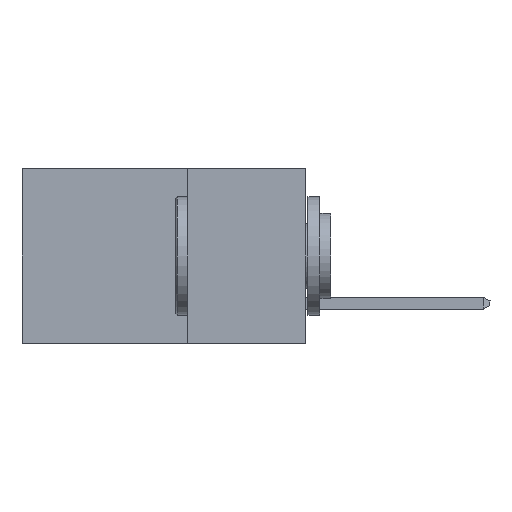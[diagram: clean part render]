
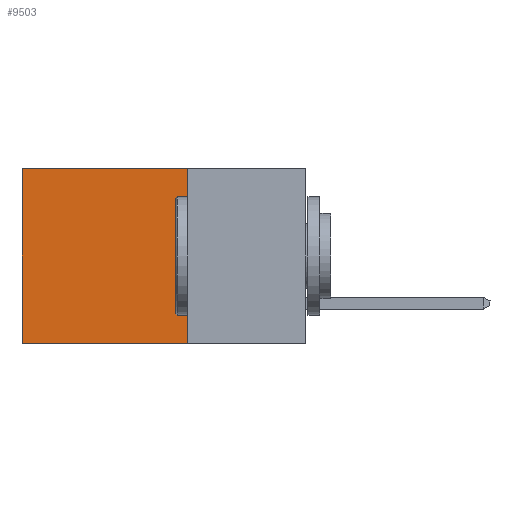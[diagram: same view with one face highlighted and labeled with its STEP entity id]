
A CAD part, left-side view. The second image highlights one B-rep face of the part: STEP entity #9503.
In plain terms, the highlighted planar face has unit normal (-1, 0, 0).
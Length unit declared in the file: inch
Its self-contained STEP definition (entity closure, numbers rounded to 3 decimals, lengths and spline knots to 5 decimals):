
#508 = EDGE_CURVE ( 'NONE', #12807, #16303, #17546, .T. ) ;
#729 = LINE ( 'NONE', #22717, #8557 ) ;
#1144 = DIRECTION ( 'NONE',  ( 1., 0., 0. ) ) ;
#1197 = ORIENTED_EDGE ( 'NONE', *, *, #27011, .F. ) ;
#1852 = CARTESIAN_POINT ( 'NONE',  ( 0.298, 0.25, 0. ) ) ;
#2166 = ORIENTED_EDGE ( 'NONE', *, *, #22689, .F. ) ;
#2172 = VECTOR ( 'NONE', #9424, 39.37008 ) ;
#3551 = CARTESIAN_POINT ( 'NONE',  ( 0.298, 0.25, 0. ) ) ;
#4534 = EDGE_LOOP ( 'NONE', ( #17804, #1197, #2166, #8695 ) ) ;
#5221 = LINE ( 'NONE', #24693, #2172 ) ;
#5830 = PLANE ( 'NONE',  #9291 ) ;
#8433 = LINE ( 'NONE', #10832, #19733 ) ;
#8557 = VECTOR ( 'NONE', #20531, 39.37008 ) ;
#8695 = ORIENTED_EDGE ( 'NONE', *, *, #508, .T. ) ;
#9291 = AXIS2_PLACEMENT_3D ( 'NONE', #3551, #1144, #12366 ) ;
#9424 = DIRECTION ( 'NONE',  ( 0., 0., -1. ) ) ;
#9503 = ADVANCED_FACE ( 'NONE', ( #22733 ), #5830, .F. ) ;
#10832 = CARTESIAN_POINT ( 'NONE',  ( 0.298, 0.25, -0.37 ) ) ;
#12366 = DIRECTION ( 'NONE',  ( 0., 0., -1. ) ) ;
#12807 = VERTEX_POINT ( 'NONE', #1852 ) ;
#16303 = VERTEX_POINT ( 'NONE', #20655 ) ;
#16926 = CARTESIAN_POINT ( 'NONE',  ( 0.298, 0.25, 0. ) ) ;
#17546 = LINE ( 'NONE', #16926, #24329 ) ;
#17804 = ORIENTED_EDGE ( 'NONE', *, *, #23942, .T. ) ;
#18317 = VERTEX_POINT ( 'NONE', #19634 ) ;
#19634 = CARTESIAN_POINT ( 'NONE',  ( 0.298, 0.6, -0.37 ) ) ;
#19733 = VECTOR ( 'NONE', #28193, 39.37008 ) ;
#20531 = DIRECTION ( 'NONE',  ( 0., 0., -1. ) ) ;
#20655 = CARTESIAN_POINT ( 'NONE',  ( 0.298, 0.6, 0. ) ) ;
#22689 = EDGE_CURVE ( 'NONE', #12807, #27379, #5221, .T. ) ;
#22717 = CARTESIAN_POINT ( 'NONE',  ( 0.298, 0.6, 0. ) ) ;
#22733 = FACE_OUTER_BOUND ( 'NONE', #4534, .T. ) ;
#23942 = EDGE_CURVE ( 'NONE', #16303, #18317, #729, .T. ) ;
#24329 = VECTOR ( 'NONE', #25659, 39.37008 ) ;
#24693 = CARTESIAN_POINT ( 'NONE',  ( 0.298, 0.25, 0. ) ) ;
#25277 = CARTESIAN_POINT ( 'NONE',  ( 0.298, 0.25, -0.37 ) ) ;
#25659 = DIRECTION ( 'NONE',  ( 0., 1., 0. ) ) ;
#27011 = EDGE_CURVE ( 'NONE', #27379, #18317, #8433, .T. ) ;
#27379 = VERTEX_POINT ( 'NONE', #25277 ) ;
#28193 = DIRECTION ( 'NONE',  ( 0., 1., 0. ) ) ;
